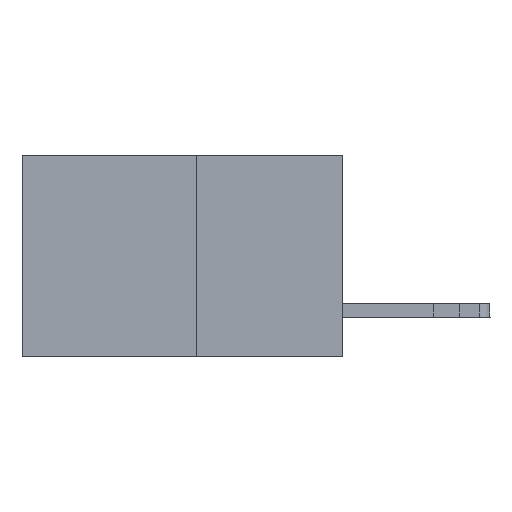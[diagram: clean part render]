
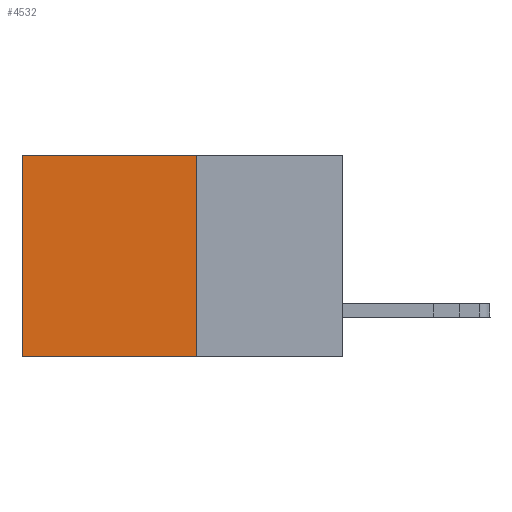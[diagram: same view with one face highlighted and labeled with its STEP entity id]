
A CAD part, left-side view. The second image highlights one B-rep face of the part: STEP entity #4532.
In plain terms, the highlighted planar face has unit normal (-1, 0, 0).
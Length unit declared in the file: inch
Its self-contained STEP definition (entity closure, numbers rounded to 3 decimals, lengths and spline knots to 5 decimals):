
#424 = VERTEX_POINT ( 'NONE', #12076 ) ;
#570 = LINE ( 'NONE', #8742, #9622 ) ;
#1424 = VERTEX_POINT ( 'NONE', #6491 ) ;
#1440 = DIRECTION ( 'NONE',  ( 0., 1., 0. ) ) ;
#1506 = EDGE_CURVE ( 'NONE', #1922, #8911, #7900, .T. ) ;
#1689 = DIRECTION ( 'NONE',  ( 0., 0., -1. ) ) ;
#1922 = VERTEX_POINT ( 'NONE', #7696 ) ;
#1973 = EDGE_CURVE ( 'NONE', #1424, #424, #3601, .T. ) ;
#2772 = ORIENTED_EDGE ( 'NONE', *, *, #10289, .F. ) ;
#2782 = CARTESIAN_POINT ( 'NONE',  ( 0.277, 0.27, -0.37 ) ) ;
#3477 = CARTESIAN_POINT ( 'NONE',  ( 0.277, 0.27, -0.37 ) ) ;
#3601 = LINE ( 'NONE', #9740, #5291 ) ;
#3696 = ORIENTED_EDGE ( 'NONE', *, *, #11098, .T. ) ;
#4261 = ORIENTED_EDGE ( 'NONE', *, *, #1506, .T. ) ;
#4532 = ADVANCED_FACE ( 'NONE', ( #10152 ), #4959, .F. ) ;
#4959 = PLANE ( 'NONE',  #12254 ) ;
#5291 = VECTOR ( 'NONE', #1689, 39.37008 ) ;
#6491 = CARTESIAN_POINT ( 'NONE',  ( 0.277, 0.27, 0. ) ) ;
#6571 = VECTOR ( 'NONE', #1440, 39.37008 ) ;
#6938 = DIRECTION ( 'NONE',  ( 1., 0., 0. ) ) ;
#7220 = ORIENTED_EDGE ( 'NONE', *, *, #1973, .F. ) ;
#7696 = CARTESIAN_POINT ( 'NONE',  ( 0.277, 0.59, 0. ) ) ;
#7725 = DIRECTION ( 'NONE',  ( 0., 1., 0. ) ) ;
#7769 = CARTESIAN_POINT ( 'NONE',  ( 0.277, 0.59, -0.37 ) ) ;
#7900 = LINE ( 'NONE', #7769, #11028 ) ;
#8656 = LINE ( 'NONE', #3477, #6571 ) ;
#8742 = CARTESIAN_POINT ( 'NONE',  ( 0.277, 0.27, 0. ) ) ;
#8911 = VERTEX_POINT ( 'NONE', #11476 ) ;
#9622 = VECTOR ( 'NONE', #7725, 39.37008 ) ;
#9740 = CARTESIAN_POINT ( 'NONE',  ( 0.277, 0.27, -0.37 ) ) ;
#10152 = FACE_OUTER_BOUND ( 'NONE', #11783, .T. ) ;
#10289 = EDGE_CURVE ( 'NONE', #424, #8911, #8656, .T. ) ;
#10911 = DIRECTION ( 'NONE',  ( 0., 0., -1. ) ) ;
#11028 = VECTOR ( 'NONE', #10911, 39.37008 ) ;
#11096 = DIRECTION ( 'NONE',  ( 0., 0., -1. ) ) ;
#11098 = EDGE_CURVE ( 'NONE', #1424, #1922, #570, .T. ) ;
#11476 = CARTESIAN_POINT ( 'NONE',  ( 0.277, 0.59, -0.37 ) ) ;
#11783 = EDGE_LOOP ( 'NONE', ( #4261, #2772, #7220, #3696 ) ) ;
#12076 = CARTESIAN_POINT ( 'NONE',  ( 0.277, 0.27, -0.37 ) ) ;
#12254 = AXIS2_PLACEMENT_3D ( 'NONE', #2782, #6938, #11096 ) ;
